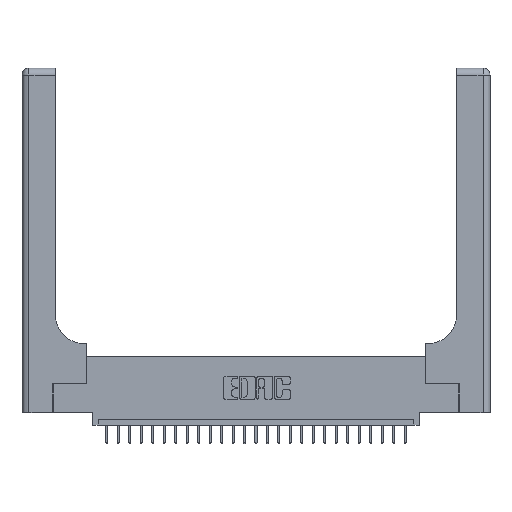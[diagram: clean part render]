
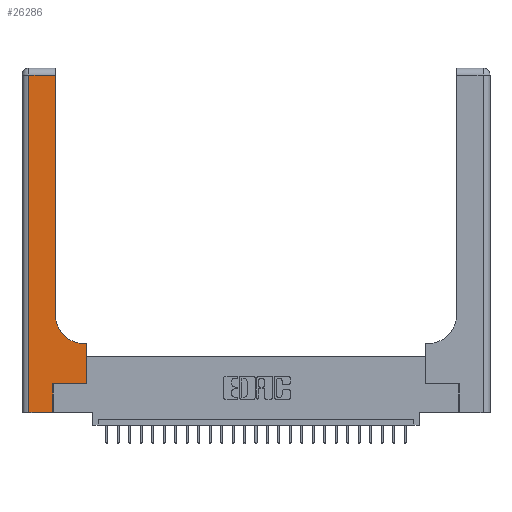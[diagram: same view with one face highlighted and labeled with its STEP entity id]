
A CAD part, top view. The second image highlights one B-rep face of the part: STEP entity #26286.
In plain terms, the highlighted planar face has unit normal (0, 0, 1).
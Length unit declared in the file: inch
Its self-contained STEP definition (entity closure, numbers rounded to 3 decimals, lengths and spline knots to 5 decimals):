
#96 = DIRECTION ( 'NONE',  ( 0., -1., 0. ) ) ;
#193 = VECTOR ( 'NONE', #20389, 39.37008 ) ;
#338 = ORIENTED_EDGE ( 'NONE', *, *, #5109, .T. ) ;
#702 = ORIENTED_EDGE ( 'NONE', *, *, #25845, .T. ) ;
#993 = DIRECTION ( 'NONE',  ( 1., 0., 0. ) ) ;
#1209 = CARTESIAN_POINT ( 'NONE',  ( 0.2915, 0.6, 0.37 ) ) ;
#1260 = LINE ( 'NONE', #1209, #19064 ) ;
#1559 = CARTESIAN_POINT ( 'NONE',  ( 0.2915, 3., 0.37 ) ) ;
#1566 = EDGE_CURVE ( 'NONE', #23606, #11688, #3117, .T. ) ;
#1749 = CARTESIAN_POINT ( 'NONE',  ( 0.2915, 0.85, 0.37 ) ) ;
#2420 = LINE ( 'NONE', #25038, #11838 ) ;
#2468 = LINE ( 'NONE', #14099, #193 ) ;
#2861 = VECTOR ( 'NONE', #26098, 39.37008 ) ;
#3117 = CIRCLE ( 'NONE', #11800, 0.25 ) ;
#3177 = ORIENTED_EDGE ( 'NONE', *, *, #15197, .T. ) ;
#3816 = EDGE_CURVE ( 'NONE', #12188, #15697, #20772, .T. ) ;
#3860 = CARTESIAN_POINT ( 'NONE',  ( 0.269, 0.25, 0.37 ) ) ;
#4267 = CARTESIAN_POINT ( 'NONE',  ( 0.06, 3., 0.37 ) ) ;
#5109 = EDGE_CURVE ( 'NONE', #15697, #19715, #2420, .T. ) ;
#5800 = CARTESIAN_POINT ( 'NONE',  ( 0.2915, 2.94, 0.37 ) ) ;
#6474 = CARTESIAN_POINT ( 'NONE',  ( 0., 2.94, 0.37 ) ) ;
#7305 = ORIENTED_EDGE ( 'NONE', *, *, #17103, .T. ) ;
#7333 = CARTESIAN_POINT ( 'NONE',  ( 0.5585, 0.25, 0.37 ) ) ;
#7442 = CARTESIAN_POINT ( 'NONE',  ( 0.5585, 0.6, 0.37 ) ) ;
#7526 = VERTEX_POINT ( 'NONE', #8414 ) ;
#7827 = EDGE_LOOP ( 'NONE', ( #14352, #7305, #3177, #23157, #338, #20784, #702, #22529, #20924 ) ) ;
#8414 = CARTESIAN_POINT ( 'NONE',  ( 0.06, 2.94, 0.37 ) ) ;
#8771 = LINE ( 'NONE', #1559, #25216 ) ;
#9897 = PLANE ( 'NONE',  #15815 ) ;
#10028 = VECTOR ( 'NONE', #12064, 39.37008 ) ;
#10444 = DIRECTION ( 'NONE',  ( -1., 0., 0. ) ) ;
#11688 = VERTEX_POINT ( 'NONE', #1749 ) ;
#11800 = AXIS2_PLACEMENT_3D ( 'NONE', #22266, #15743, #993 ) ;
#11838 = VECTOR ( 'NONE', #16638, 39.37008 ) ;
#11976 = CARTESIAN_POINT ( 'NONE',  ( 0., 3., 0.37 ) ) ;
#12064 = DIRECTION ( 'NONE',  ( 1., 0., 0. ) ) ;
#12188 = VERTEX_POINT ( 'NONE', #13888 ) ;
#12895 = EDGE_CURVE ( 'NONE', #11688, #26978, #8771, .T. ) ;
#12949 = FACE_OUTER_BOUND ( 'NONE', #7827, .T. ) ;
#13888 = CARTESIAN_POINT ( 'NONE',  ( 0.06, 0., 0.37 ) ) ;
#13966 = DIRECTION ( 'NONE',  ( -1., 0., 0. ) ) ;
#14005 = VECTOR ( 'NONE', #96, 39.37008 ) ;
#14099 = CARTESIAN_POINT ( 'NONE',  ( 0.269, 0.25, 0.37 ) ) ;
#14352 = ORIENTED_EDGE ( 'NONE', *, *, #12895, .T. ) ;
#14489 = CARTESIAN_POINT ( 'NONE',  ( 0., 0., 0.37 ) ) ;
#15197 = EDGE_CURVE ( 'NONE', #7526, #12188, #20388, .T. ) ;
#15598 = LINE ( 'NONE', #6474, #19934 ) ;
#15697 = VERTEX_POINT ( 'NONE', #17378 ) ;
#15743 = DIRECTION ( 'NONE',  ( 0., 0., -1. ) ) ;
#15815 = AXIS2_PLACEMENT_3D ( 'NONE', #11976, #26958, #24812 ) ;
#16638 = DIRECTION ( 'NONE',  ( 0., 1., 0. ) ) ;
#16797 = EDGE_CURVE ( 'NONE', #19715, #16855, #2468, .T. ) ;
#16855 = VERTEX_POINT ( 'NONE', #7333 ) ;
#17103 = EDGE_CURVE ( 'NONE', #26978, #7526, #15598, .T. ) ;
#17378 = CARTESIAN_POINT ( 'NONE',  ( 0.269, 0., 0.37 ) ) ;
#18103 = CARTESIAN_POINT ( 'NONE',  ( 0.5415, 0.6, 0.37 ) ) ;
#19064 = VECTOR ( 'NONE', #13966, 39.37008 ) ;
#19327 = LINE ( 'NONE', #23853, #2861 ) ;
#19715 = VERTEX_POINT ( 'NONE', #3860 ) ;
#19934 = VECTOR ( 'NONE', #10444, 39.37008 ) ;
#20388 = LINE ( 'NONE', #4267, #14005 ) ;
#20389 = DIRECTION ( 'NONE',  ( 1., 0., 0. ) ) ;
#20772 = LINE ( 'NONE', #14489, #10028 ) ;
#20784 = ORIENTED_EDGE ( 'NONE', *, *, #16797, .T. ) ;
#20924 = ORIENTED_EDGE ( 'NONE', *, *, #1566, .T. ) ;
#22266 = CARTESIAN_POINT ( 'NONE',  ( 0.5415, 0.85, 0.37 ) ) ;
#22529 = ORIENTED_EDGE ( 'NONE', *, *, #24854, .T. ) ;
#23157 = ORIENTED_EDGE ( 'NONE', *, *, #3816, .T. ) ;
#23606 = VERTEX_POINT ( 'NONE', #18103 ) ;
#23853 = CARTESIAN_POINT ( 'NONE',  ( 0.5585, 0.25, 0.37 ) ) ;
#24812 = DIRECTION ( 'NONE',  ( -1., 0., 0. ) ) ;
#24854 = EDGE_CURVE ( 'NONE', #25537, #23606, #1260, .T. ) ;
#25038 = CARTESIAN_POINT ( 'NONE',  ( 0.269, 0., 0.37 ) ) ;
#25216 = VECTOR ( 'NONE', #25275, 39.37008 ) ;
#25275 = DIRECTION ( 'NONE',  ( 0., 1., 0. ) ) ;
#25537 = VERTEX_POINT ( 'NONE', #7442 ) ;
#25845 = EDGE_CURVE ( 'NONE', #16855, #25537, #19327, .T. ) ;
#26098 = DIRECTION ( 'NONE',  ( 0., 1., 0. ) ) ;
#26286 = ADVANCED_FACE ( 'NONE', ( #12949 ), #9897, .F. ) ;
#26958 = DIRECTION ( 'NONE',  ( 0., 0., -1. ) ) ;
#26978 = VERTEX_POINT ( 'NONE', #5800 ) ;
